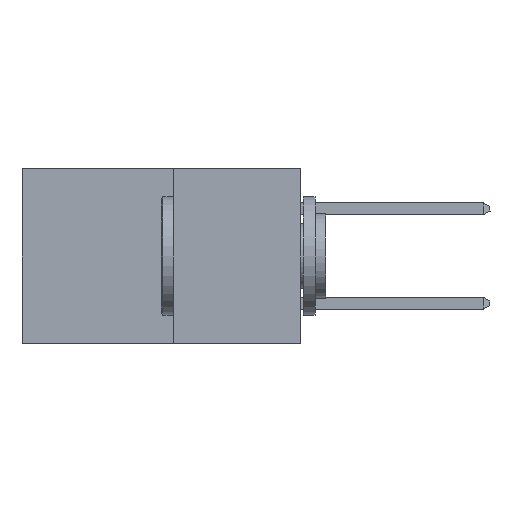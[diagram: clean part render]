
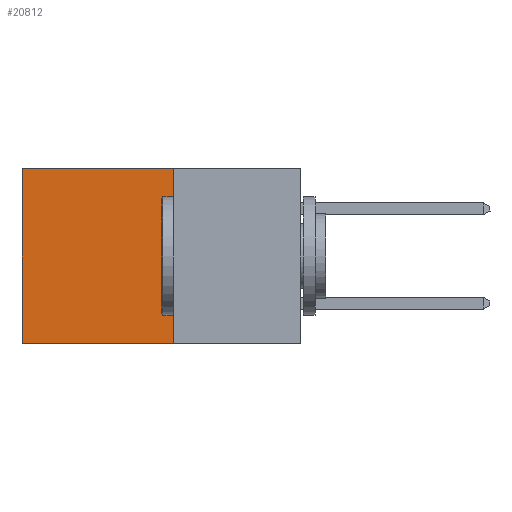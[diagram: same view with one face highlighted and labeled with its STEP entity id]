
A CAD part, left-side view. The second image highlights one B-rep face of the part: STEP entity #20812.
In plain terms, the highlighted planar face has unit normal (-1, 0, 0).
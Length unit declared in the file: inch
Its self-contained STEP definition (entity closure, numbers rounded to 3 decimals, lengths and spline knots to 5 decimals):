
#879 = VERTEX_POINT ( 'NONE', #19247 ) ;
#2028 = DIRECTION ( 'NONE',  ( 0., 0., -1. ) ) ;
#2169 = VERTEX_POINT ( 'NONE', #5872 ) ;
#2441 = CARTESIAN_POINT ( 'NONE',  ( 0.277, 0.27, -0.37 ) ) ;
#4820 = LINE ( 'NONE', #18504, #25485 ) ;
#5148 = DIRECTION ( 'NONE',  ( 0., 0., -1. ) ) ;
#5297 = VECTOR ( 'NONE', #2028, 39.37008 ) ;
#5872 = CARTESIAN_POINT ( 'NONE',  ( 0.277, 0.59, 0. ) ) ;
#5926 = EDGE_LOOP ( 'NONE', ( #17456, #29425, #31936, #10486 ) ) ;
#7481 = VERTEX_POINT ( 'NONE', #9964 ) ;
#9778 = FACE_OUTER_BOUND ( 'NONE', #5926, .T. ) ;
#9964 = CARTESIAN_POINT ( 'NONE',  ( 0.277, 0.27, 0. ) ) ;
#10486 = ORIENTED_EDGE ( 'NONE', *, *, #17402, .T. ) ;
#11102 = DIRECTION ( 'NONE',  ( 0., 1., 0. ) ) ;
#13686 = CARTESIAN_POINT ( 'NONE',  ( 0.277, 0.27, 0. ) ) ;
#15005 = CARTESIAN_POINT ( 'NONE',  ( 0.277, 0.27, -0.37 ) ) ;
#15398 = PLANE ( 'NONE',  #18735 ) ;
#17402 = EDGE_CURVE ( 'NONE', #7481, #2169, #31185, .T. ) ;
#17456 = ORIENTED_EDGE ( 'NONE', *, *, #31977, .T. ) ;
#18477 = VECTOR ( 'NONE', #33757, 39.37008 ) ;
#18504 = CARTESIAN_POINT ( 'NONE',  ( 0.277, 0.27, -0.37 ) ) ;
#18735 = AXIS2_PLACEMENT_3D ( 'NONE', #2441, #21331, #5148 ) ;
#19247 = CARTESIAN_POINT ( 'NONE',  ( 0.277, 0.27, -0.37 ) ) ;
#19635 = EDGE_CURVE ( 'NONE', #879, #31598, #4820, .T. ) ;
#20812 = ADVANCED_FACE ( 'NONE', ( #9778 ), #15398, .F. ) ;
#21331 = DIRECTION ( 'NONE',  ( 1., 0., 0. ) ) ;
#21720 = DIRECTION ( 'NONE',  ( 0., 1., 0. ) ) ;
#23429 = EDGE_CURVE ( 'NONE', #7481, #879, #32687, .T. ) ;
#23588 = CARTESIAN_POINT ( 'NONE',  ( 0.277, 0.59, -0.37 ) ) ;
#24117 = VECTOR ( 'NONE', #11102, 39.37008 ) ;
#25485 = VECTOR ( 'NONE', #21720, 39.37008 ) ;
#29425 = ORIENTED_EDGE ( 'NONE', *, *, #19635, .F. ) ;
#30254 = CARTESIAN_POINT ( 'NONE',  ( 0.277, 0.59, -0.37 ) ) ;
#31185 = LINE ( 'NONE', #13686, #24117 ) ;
#31598 = VERTEX_POINT ( 'NONE', #30254 ) ;
#31936 = ORIENTED_EDGE ( 'NONE', *, *, #23429, .F. ) ;
#31977 = EDGE_CURVE ( 'NONE', #2169, #31598, #33030, .T. ) ;
#32687 = LINE ( 'NONE', #15005, #18477 ) ;
#33030 = LINE ( 'NONE', #23588, #5297 ) ;
#33757 = DIRECTION ( 'NONE',  ( 0., 0., -1. ) ) ;
